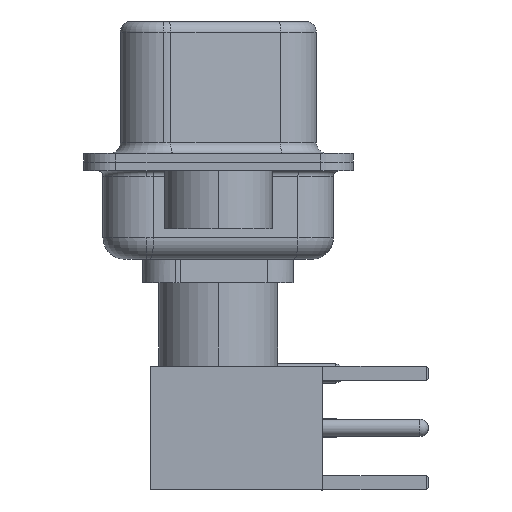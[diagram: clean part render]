
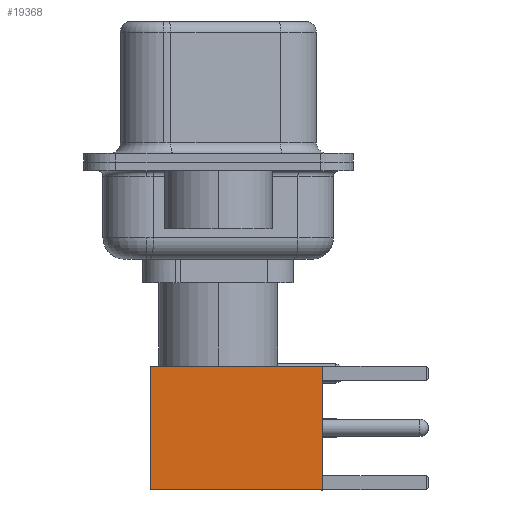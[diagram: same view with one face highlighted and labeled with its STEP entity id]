
A CAD part, left-side view. The second image highlights one B-rep face of the part: STEP entity #19368.
In plain terms, the highlighted face is planar.
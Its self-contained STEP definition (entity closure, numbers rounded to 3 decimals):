
#48 = ORIENTED_EDGE ( 'NONE', *, *, #17594, .F. ) ;
#474 = DIRECTION ( 'NONE',  ( 0., 0., -1. ) ) ;
#558 = DIRECTION ( 'NONE',  ( 0., 1., 0. ) ) ;
#2186 = ORIENTED_EDGE ( 'NONE', *, *, #3989, .T. ) ;
#3244 = VERTEX_POINT ( 'NONE', #5566 ) ;
#3858 = AXIS2_PLACEMENT_3D ( 'NONE', #15562, #558, #4276 ) ;
#3989 = EDGE_CURVE ( 'NONE', #3244, #23257, #13783, .T. ) ;
#4276 = DIRECTION ( 'NONE',  ( 0., 0., 1. ) ) ;
#5566 = CARTESIAN_POINT ( 'NONE',  ( 2.875, 2.875, 0. ) ) ;
#7605 = ORIENTED_EDGE ( 'NONE', *, *, #15978, .F. ) ;
#8382 = CARTESIAN_POINT ( 'NONE',  ( 2.875, 2.875, 8. ) ) ;
#8582 = VECTOR ( 'NONE', #20663, 1000. ) ;
#8851 = PLANE ( 'NONE',  #3858 ) ;
#9003 = VERTEX_POINT ( 'NONE', #8382 ) ;
#9271 = FACE_OUTER_BOUND ( 'NONE', #26533, .T. ) ;
#10697 = LINE ( 'NONE', #19424, #8582 ) ;
#11145 = VECTOR ( 'NONE', #474, 1000. ) ;
#11221 = DIRECTION ( 'NONE',  ( -1., 0., 0. ) ) ;
#12594 = CARTESIAN_POINT ( 'NONE',  ( -2.875, 2.875, 8. ) ) ;
#13783 = LINE ( 'NONE', #22082, #23280 ) ;
#13799 = ORIENTED_EDGE ( 'NONE', *, *, #22590, .T. ) ;
#15562 = CARTESIAN_POINT ( 'NONE',  ( 2.875, 2.875, 0. ) ) ;
#15978 = EDGE_CURVE ( 'NONE', #9003, #17990, #20222, .T. ) ;
#16079 = CARTESIAN_POINT ( 'NONE',  ( 0., 2.875, 8. ) ) ;
#17594 = EDGE_CURVE ( 'NONE', #17990, #23257, #26618, .T. ) ;
#17934 = VECTOR ( 'NONE', #24783, 1000. ) ;
#17990 = VERTEX_POINT ( 'NONE', #12594 ) ;
#19368 = ADVANCED_FACE ( 'NONE', ( #9271 ), #8851, .T. ) ;
#19424 = CARTESIAN_POINT ( 'NONE',  ( 2.875, 2.875, 0. ) ) ;
#20222 = LINE ( 'NONE', #16079, #17934 ) ;
#20663 = DIRECTION ( 'NONE',  ( 0., 0., -1. ) ) ;
#21909 = CARTESIAN_POINT ( 'NONE',  ( -2.875, 2.875, 0. ) ) ;
#22082 = CARTESIAN_POINT ( 'NONE',  ( 0., 2.875, 0. ) ) ;
#22590 = EDGE_CURVE ( 'NONE', #9003, #3244, #10697, .T. ) ;
#23257 = VERTEX_POINT ( 'NONE', #28218 ) ;
#23280 = VECTOR ( 'NONE', #11221, 1000. ) ;
#24783 = DIRECTION ( 'NONE',  ( -1., 0., 0. ) ) ;
#26533 = EDGE_LOOP ( 'NONE', ( #13799, #2186, #48, #7605 ) ) ;
#26618 = LINE ( 'NONE', #21909, #11145 ) ;
#28218 = CARTESIAN_POINT ( 'NONE',  ( -2.875, 2.875, 0. ) ) ;
